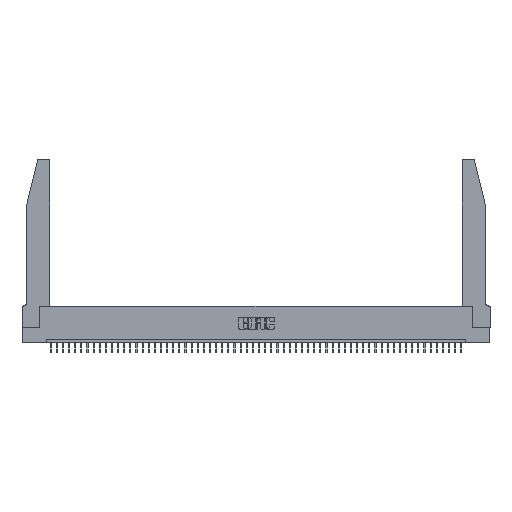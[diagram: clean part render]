
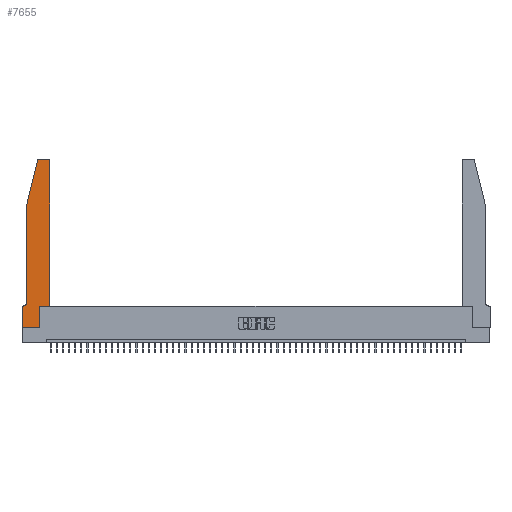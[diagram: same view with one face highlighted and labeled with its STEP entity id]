
A CAD part, top view. The second image highlights one B-rep face of the part: STEP entity #7655.
In plain terms, the highlighted planar face has unit normal (0, 0, 1).
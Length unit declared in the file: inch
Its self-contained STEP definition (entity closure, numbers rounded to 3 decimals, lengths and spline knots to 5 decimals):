
#117 = ORIENTED_EDGE ( 'NONE', *, *, #209, .T. ) ;
#209 = EDGE_CURVE ( 'NONE', #44470, #10463, #7759, .T. ) ;
#211 = DIRECTION ( 'NONE',  ( 1., 0., 0. ) ) ;
#590 = EDGE_CURVE ( 'NONE', #10150, #25188, #12736, .T. ) ;
#1293 = VECTOR ( 'NONE', #17419, 39.37008 ) ;
#1702 = DIRECTION ( 'NONE',  ( -1., 0., 0. ) ) ;
#2066 = CARTESIAN_POINT ( 'NONE',  ( 0., 0.35, 0.37 ) ) ;
#3879 = VECTOR ( 'NONE', #4621, 39.37008 ) ;
#4529 = VERTEX_POINT ( 'NONE', #37021 ) ;
#4621 = DIRECTION ( 'NONE',  ( 0., -1., 0. ) ) ;
#5709 = LINE ( 'NONE', #11464, #36809 ) ;
#5874 = EDGE_LOOP ( 'NONE', ( #16708, #23961, #8952, #29673, #35525, #33292, #29223, #38866, #40947, #24867, #117, #35583 ) ) ;
#5998 = EDGE_CURVE ( 'NONE', #12613, #29780, #13353, .T. ) ;
#6009 = CARTESIAN_POINT ( 'NONE',  ( 0.0055, 0.42, 0.37 ) ) ;
#6213 = FACE_OUTER_BOUND ( 'NONE', #5874, .T. ) ;
#7655 = ADVANCED_FACE ( 'NONE', ( #6213 ), #47253, .T. ) ;
#7759 = LINE ( 'NONE', #13580, #36905 ) ;
#8050 = VERTEX_POINT ( 'NONE', #44264 ) ;
#8952 = ORIENTED_EDGE ( 'NONE', *, *, #9768, .T. ) ;
#9768 = EDGE_CURVE ( 'NONE', #25188, #12613, #46541, .T. ) ;
#10150 = VERTEX_POINT ( 'NONE', #34545 ) ;
#10463 = VERTEX_POINT ( 'NONE', #34522 ) ;
#10626 = DIRECTION ( 'NONE',  ( 1., 0., 0. ) ) ;
#11094 = VERTEX_POINT ( 'NONE', #34873 ) ;
#11464 = CARTESIAN_POINT ( 'NONE',  ( 0.2605, 2.75, 0.37 ) ) ;
#11509 = CARTESIAN_POINT ( 'NONE',  ( 0.0755, 2., 0.37 ) ) ;
#12613 = VERTEX_POINT ( 'NONE', #11509 ) ;
#12732 = LINE ( 'NONE', #22600, #35621 ) ;
#12736 = CIRCLE ( 'NONE', #30301, 0.03 ) ;
#12860 = DIRECTION ( 'NONE',  ( 1., 0., 0. ) ) ;
#13353 = LINE ( 'NONE', #41689, #3879 ) ;
#13580 = CARTESIAN_POINT ( 'NONE',  ( 0.4505, 0.35, 0.37 ) ) ;
#14218 = EDGE_CURVE ( 'NONE', #40354, #4529, #52291, .T. ) ;
#15615 = CARTESIAN_POINT ( 'NONE',  ( 0., 0.35, 0.37 ) ) ;
#15624 = EDGE_CURVE ( 'NONE', #8050, #42002, #48864, .T. ) ;
#15845 = EDGE_CURVE ( 'NONE', #18945, #40354, #12732, .T. ) ;
#16708 = ORIENTED_EDGE ( 'NONE', *, *, #24306, .T. ) ;
#17419 = DIRECTION ( 'NONE',  ( 0., 1., 0. ) ) ;
#18945 = VERTEX_POINT ( 'NONE', #45796 ) ;
#19468 = CARTESIAN_POINT ( 'NONE',  ( 0.2865, 0.35, 0.37 ) ) ;
#21890 = DIRECTION ( 'NONE',  ( -1., 0., 0. ) ) ;
#22474 = CARTESIAN_POINT ( 'NONE',  ( 0., 0., 0.37 ) ) ;
#22486 = LINE ( 'NONE', #40214, #36385 ) ;
#22600 = CARTESIAN_POINT ( 'NONE',  ( 0.0755, 0.35, 0.37 ) ) ;
#22622 = DIRECTION ( 'NONE',  ( 0., 0., 1. ) ) ;
#23149 = DIRECTION ( 'NONE',  ( 0., -1., 0. ) ) ;
#23961 = ORIENTED_EDGE ( 'NONE', *, *, #590, .T. ) ;
#24306 = EDGE_CURVE ( 'NONE', #11094, #10150, #5709, .T. ) ;
#24867 = ORIENTED_EDGE ( 'NONE', *, *, #43313, .T. ) ;
#25188 = VERTEX_POINT ( 'NONE', #36778 ) ;
#25276 = CARTESIAN_POINT ( 'NONE',  ( 0.284, 2.72, 0.37 ) ) ;
#25819 = DIRECTION ( 'NONE',  ( 0., 0., 1. ) ) ;
#27608 = CARTESIAN_POINT ( 'NONE',  ( 0., 0., 0.37 ) ) ;
#28347 = EDGE_CURVE ( 'NONE', #29780, #18945, #34483, .T. ) ;
#29223 = ORIENTED_EDGE ( 'NONE', *, *, #14218, .T. ) ;
#29663 = CARTESIAN_POINT ( 'NONE',  ( 0.0755, 0.42, 0.37 ) ) ;
#29673 = ORIENTED_EDGE ( 'NONE', *, *, #5998, .T. ) ;
#29780 = VERTEX_POINT ( 'NONE', #29663 ) ;
#30301 = AXIS2_PLACEMENT_3D ( 'NONE', #25276, #25819, #50253 ) ;
#30740 = LINE ( 'NONE', #22474, #38964 ) ;
#33292 = ORIENTED_EDGE ( 'NONE', *, *, #15845, .T. ) ;
#33849 = VECTOR ( 'NONE', #23149, 39.37008 ) ;
#34483 = CIRCLE ( 'NONE', #39396, 0.07 ) ;
#34522 = CARTESIAN_POINT ( 'NONE',  ( 0.4505, 2.72, 0.37 ) ) ;
#34545 = CARTESIAN_POINT ( 'NONE',  ( 0.284, 2.75, 0.37 ) ) ;
#34873 = CARTESIAN_POINT ( 'NONE',  ( 0.4205, 2.75, 0.37 ) ) ;
#35525 = ORIENTED_EDGE ( 'NONE', *, *, #28347, .T. ) ;
#35583 = ORIENTED_EDGE ( 'NONE', *, *, #44062, .T. ) ;
#35621 = VECTOR ( 'NONE', #21890, 39.37008 ) ;
#36172 = CIRCLE ( 'NONE', #52438, 0.03 ) ;
#36318 = DIRECTION ( 'NONE',  ( 1., 0., 0. ) ) ;
#36385 = VECTOR ( 'NONE', #36318, 39.37008 ) ;
#36778 = CARTESIAN_POINT ( 'NONE',  ( 0.25487, 2.72718, 0.37 ) ) ;
#36809 = VECTOR ( 'NONE', #40163, 39.37008 ) ;
#36905 = VECTOR ( 'NONE', #37867, 39.37008 ) ;
#37021 = CARTESIAN_POINT ( 'NONE',  ( 0., 0., 0.37 ) ) ;
#37867 = DIRECTION ( 'NONE',  ( 0., 1., 0. ) ) ;
#38087 = DIRECTION ( 'NONE',  ( 0., 0., -1. ) ) ;
#38866 = ORIENTED_EDGE ( 'NONE', *, *, #40267, .T. ) ;
#38964 = VECTOR ( 'NONE', #10626, 39.37008 ) ;
#39396 = AXIS2_PLACEMENT_3D ( 'NONE', #6009, #38087, #1702 ) ;
#39524 = CARTESIAN_POINT ( 'NONE',  ( 0.0755, 2., 0.37 ) ) ;
#40163 = DIRECTION ( 'NONE',  ( -1., 0., 0. ) ) ;
#40214 = CARTESIAN_POINT ( 'NONE',  ( 0.4505, 0.35, 0.37 ) ) ;
#40267 = EDGE_CURVE ( 'NONE', #4529, #8050, #30740, .T. ) ;
#40354 = VERTEX_POINT ( 'NONE', #15615 ) ;
#40810 = DIRECTION ( 'NONE',  ( 0., 0., 1. ) ) ;
#40890 = VECTOR ( 'NONE', #42848, 39.37008 ) ;
#40947 = ORIENTED_EDGE ( 'NONE', *, *, #15624, .T. ) ;
#41689 = CARTESIAN_POINT ( 'NONE',  ( 0.0755, 2., 0.37 ) ) ;
#42002 = VERTEX_POINT ( 'NONE', #19468 ) ;
#42676 = AXIS2_PLACEMENT_3D ( 'NONE', #2066, #22622, #12860 ) ;
#42848 = DIRECTION ( 'NONE',  ( -0.239, -0.971, 0. ) ) ;
#43313 = EDGE_CURVE ( 'NONE', #42002, #44470, #22486, .T. ) ;
#44062 = EDGE_CURVE ( 'NONE', #10463, #11094, #36172, .T. ) ;
#44264 = CARTESIAN_POINT ( 'NONE',  ( 0.2865, 0., 0.37 ) ) ;
#44470 = VERTEX_POINT ( 'NONE', #52147 ) ;
#45796 = CARTESIAN_POINT ( 'NONE',  ( 0.0055, 0.35, 0.37 ) ) ;
#46194 = CARTESIAN_POINT ( 'NONE',  ( 0.2865, 0.35, 0.37 ) ) ;
#46541 = LINE ( 'NONE', #39524, #40890 ) ;
#47253 = PLANE ( 'NONE',  #42676 ) ;
#48600 = CARTESIAN_POINT ( 'NONE',  ( 0.4205, 2.72, 0.37 ) ) ;
#48864 = LINE ( 'NONE', #46194, #1293 ) ;
#50253 = DIRECTION ( 'NONE',  ( 1., 0., 0. ) ) ;
#52147 = CARTESIAN_POINT ( 'NONE',  ( 0.4505, 0.35, 0.37 ) ) ;
#52291 = LINE ( 'NONE', #27608, #33849 ) ;
#52438 = AXIS2_PLACEMENT_3D ( 'NONE', #48600, #40810, #211 ) ;
